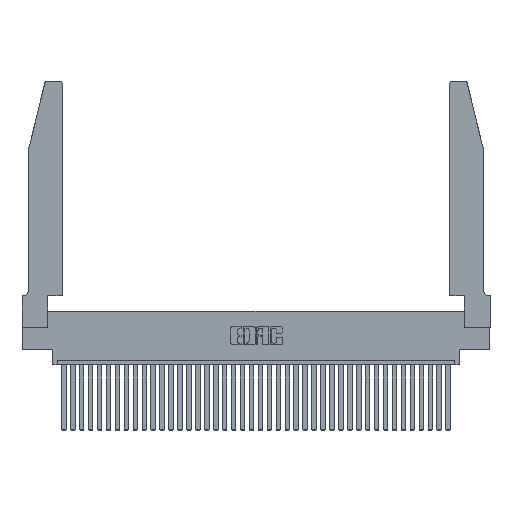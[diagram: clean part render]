
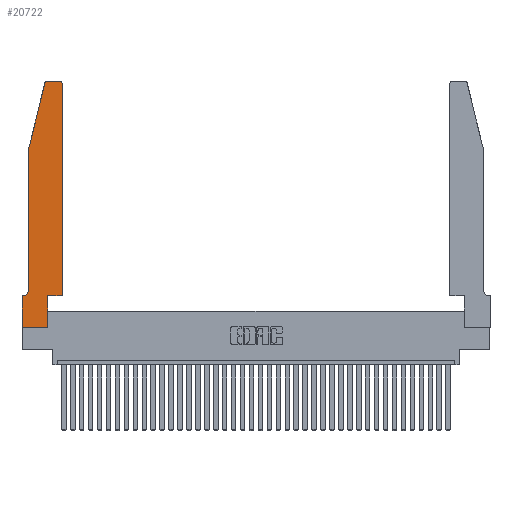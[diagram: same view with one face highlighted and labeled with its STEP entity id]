
A CAD part, top view. The second image highlights one B-rep face of the part: STEP entity #20722.
In plain terms, the highlighted planar face has unit normal (0, 0, 1).
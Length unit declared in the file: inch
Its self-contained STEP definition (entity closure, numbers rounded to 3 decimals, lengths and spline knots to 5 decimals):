
#205 = DIRECTION ( 'NONE',  ( 0., -1., 0. ) ) ;
#247 = VECTOR ( 'NONE', #18984, 39.37008 ) ;
#519 = VECTOR ( 'NONE', #31377, 39.37008 ) ;
#1791 = DIRECTION ( 'NONE',  ( 1., 0., 0. ) ) ;
#2365 = ORIENTED_EDGE ( 'NONE', *, *, #12951, .T. ) ;
#3295 = EDGE_CURVE ( 'NONE', #16624, #21802, #6180, .T. ) ;
#3690 = VERTEX_POINT ( 'NONE', #7696 ) ;
#3777 = EDGE_CURVE ( 'NONE', #16134, #16624, #28448, .T. ) ;
#4369 = ORIENTED_EDGE ( 'NONE', *, *, #4507, .T. ) ;
#4507 = EDGE_CURVE ( 'NONE', #34466, #29771, #30644, .T. ) ;
#4843 = EDGE_CURVE ( 'NONE', #34235, #20024, #15168, .T. ) ;
#5277 = DIRECTION ( 'NONE',  ( -0.239, -0.971, 0. ) ) ;
#5660 = CARTESIAN_POINT ( 'NONE',  ( 0.25487, 2.72718, 0.37 ) ) ;
#5789 = ORIENTED_EDGE ( 'NONE', *, *, #15456, .T. ) ;
#6180 = LINE ( 'NONE', #20692, #12575 ) ;
#7357 = VECTOR ( 'NONE', #10243, 39.37008 ) ;
#7696 = CARTESIAN_POINT ( 'NONE',  ( 0.2865, 0., 0.37 ) ) ;
#8141 = CARTESIAN_POINT ( 'NONE',  ( 0.4505, 0.35, 0.37 ) ) ;
#8478 = ORIENTED_EDGE ( 'NONE', *, *, #12542, .T. ) ;
#8930 = CARTESIAN_POINT ( 'NONE',  ( 0., 0.35, 0.37 ) ) ;
#8931 = ORIENTED_EDGE ( 'NONE', *, *, #23964, .T. ) ;
#9040 = DIRECTION ( 'NONE',  ( -1., 0., 0. ) ) ;
#9819 = AXIS2_PLACEMENT_3D ( 'NONE', #24844, #33517, #1791 ) ;
#9960 = CARTESIAN_POINT ( 'NONE',  ( 0.2605, 2.75, 0.37 ) ) ;
#10243 = DIRECTION ( 'NONE',  ( 1., 0., 0. ) ) ;
#10736 = VECTOR ( 'NONE', #5277, 39.37008 ) ;
#10779 = ORIENTED_EDGE ( 'NONE', *, *, #3777, .T. ) ;
#11131 = VECTOR ( 'NONE', #12914, 39.37008 ) ;
#11503 = CARTESIAN_POINT ( 'NONE',  ( 0.0755, 2., 0.37 ) ) ;
#11596 = CARTESIAN_POINT ( 'NONE',  ( 0.284, 2.75, 0.37 ) ) ;
#11915 = CARTESIAN_POINT ( 'NONE',  ( 0.2865, 0.35, 0.37 ) ) ;
#12224 = CARTESIAN_POINT ( 'NONE',  ( 0.2865, 0.35, 0.37 ) ) ;
#12542 = EDGE_CURVE ( 'NONE', #3690, #18731, #31491, .T. ) ;
#12575 = VECTOR ( 'NONE', #205, 39.37008 ) ;
#12914 = DIRECTION ( 'NONE',  ( -1., 0., 0. ) ) ;
#12951 = EDGE_CURVE ( 'NONE', #29771, #16134, #32325, .T. ) ;
#13249 = PLANE ( 'NONE',  #9819 ) ;
#13714 = CARTESIAN_POINT ( 'NONE',  ( 0.4505, 0.35, 0.37 ) ) ;
#14049 = CARTESIAN_POINT ( 'NONE',  ( 0.4205, 2.72, 0.37 ) ) ;
#14190 = DIRECTION ( 'NONE',  ( -1., 0., 0. ) ) ;
#14712 = EDGE_CURVE ( 'NONE', #20024, #32909, #15655, .T. ) ;
#15163 = CARTESIAN_POINT ( 'NONE',  ( 0.0055, 0.42, 0.37 ) ) ;
#15168 = LINE ( 'NONE', #31306, #22939 ) ;
#15279 = EDGE_CURVE ( 'NONE', #18394, #23338, #25617, .T. ) ;
#15376 = ORIENTED_EDGE ( 'NONE', *, *, #28176, .T. ) ;
#15456 = EDGE_CURVE ( 'NONE', #32909, #3690, #34580, .T. ) ;
#15525 = ORIENTED_EDGE ( 'NONE', *, *, #14712, .T. ) ;
#15542 = DIRECTION ( 'NONE',  ( 1., 0., 0. ) ) ;
#15592 = VECTOR ( 'NONE', #35778, 39.37008 ) ;
#15655 = LINE ( 'NONE', #19056, #17462 ) ;
#16134 = VERTEX_POINT ( 'NONE', #5660 ) ;
#16269 = DIRECTION ( 'NONE',  ( 0., -1., 0. ) ) ;
#16624 = VERTEX_POINT ( 'NONE', #36129 ) ;
#17462 = VECTOR ( 'NONE', #16269, 39.37008 ) ;
#17879 = AXIS2_PLACEMENT_3D ( 'NONE', #26705, #26352, #15542 ) ;
#18062 = CARTESIAN_POINT ( 'NONE',  ( 0.0755, 0.42, 0.37 ) ) ;
#18394 = VERTEX_POINT ( 'NONE', #13714 ) ;
#18650 = AXIS2_PLACEMENT_3D ( 'NONE', #14049, #28507, #25737 ) ;
#18731 = VERTEX_POINT ( 'NONE', #11915 ) ;
#18780 = CARTESIAN_POINT ( 'NONE',  ( 0., 0., 0.37 ) ) ;
#18984 = DIRECTION ( 'NONE',  ( 1., 0., 0. ) ) ;
#19056 = CARTESIAN_POINT ( 'NONE',  ( 0., 0., 0.37 ) ) ;
#20024 = VERTEX_POINT ( 'NONE', #8930 ) ;
#20692 = CARTESIAN_POINT ( 'NONE',  ( 0.0755, 2., 0.37 ) ) ;
#20722 = ADVANCED_FACE ( 'NONE', ( #31329 ), #13249, .T. ) ;
#21256 = AXIS2_PLACEMENT_3D ( 'NONE', #15163, #32630, #9040 ) ;
#21802 = VERTEX_POINT ( 'NONE', #18062 ) ;
#21854 = CIRCLE ( 'NONE', #21256, 0.07 ) ;
#22939 = VECTOR ( 'NONE', #14190, 39.37008 ) ;
#23338 = VERTEX_POINT ( 'NONE', #30937 ) ;
#23964 = EDGE_CURVE ( 'NONE', #23338, #34466, #24258, .T. ) ;
#24258 = CIRCLE ( 'NONE', #18650, 0.03 ) ;
#24424 = LINE ( 'NONE', #24580, #247 ) ;
#24580 = CARTESIAN_POINT ( 'NONE',  ( 0.4505, 0.35, 0.37 ) ) ;
#24844 = CARTESIAN_POINT ( 'NONE',  ( 0., 0.35, 0.37 ) ) ;
#25617 = LINE ( 'NONE', #8141, #519 ) ;
#25737 = DIRECTION ( 'NONE',  ( 1., 0., 0. ) ) ;
#26352 = DIRECTION ( 'NONE',  ( 0., 0., 1. ) ) ;
#26705 = CARTESIAN_POINT ( 'NONE',  ( 0.284, 2.72, 0.37 ) ) ;
#28176 = EDGE_CURVE ( 'NONE', #18731, #18394, #24424, .T. ) ;
#28448 = LINE ( 'NONE', #11503, #10736 ) ;
#28507 = DIRECTION ( 'NONE',  ( 0., 0., 1. ) ) ;
#28786 = ORIENTED_EDGE ( 'NONE', *, *, #3295, .T. ) ;
#28847 = ORIENTED_EDGE ( 'NONE', *, *, #15279, .T. ) ;
#29771 = VERTEX_POINT ( 'NONE', #11596 ) ;
#30644 = LINE ( 'NONE', #9960, #11131 ) ;
#30937 = CARTESIAN_POINT ( 'NONE',  ( 0.4505, 2.72, 0.37 ) ) ;
#31306 = CARTESIAN_POINT ( 'NONE',  ( 0.0755, 0.35, 0.37 ) ) ;
#31329 = FACE_OUTER_BOUND ( 'NONE', #32513, .T. ) ;
#31377 = DIRECTION ( 'NONE',  ( 0., 1., 0. ) ) ;
#31491 = LINE ( 'NONE', #12224, #15592 ) ;
#31968 = EDGE_CURVE ( 'NONE', #21802, #34235, #21854, .T. ) ;
#32325 = CIRCLE ( 'NONE', #17879, 0.03 ) ;
#32513 = EDGE_LOOP ( 'NONE', ( #4369, #2365, #10779, #28786, #34393, #33490, #15525, #5789, #8478, #15376, #28847, #8931 ) ) ;
#32630 = DIRECTION ( 'NONE',  ( 0., 0., -1. ) ) ;
#32909 = VERTEX_POINT ( 'NONE', #35187 ) ;
#33490 = ORIENTED_EDGE ( 'NONE', *, *, #4843, .T. ) ;
#33517 = DIRECTION ( 'NONE',  ( 0., 0., 1. ) ) ;
#34083 = CARTESIAN_POINT ( 'NONE',  ( 0.0055, 0.35, 0.37 ) ) ;
#34235 = VERTEX_POINT ( 'NONE', #34083 ) ;
#34393 = ORIENTED_EDGE ( 'NONE', *, *, #31968, .T. ) ;
#34466 = VERTEX_POINT ( 'NONE', #37450 ) ;
#34580 = LINE ( 'NONE', #18780, #7357 ) ;
#35187 = CARTESIAN_POINT ( 'NONE',  ( 0., 0., 0.37 ) ) ;
#35778 = DIRECTION ( 'NONE',  ( 0., 1., 0. ) ) ;
#36129 = CARTESIAN_POINT ( 'NONE',  ( 0.0755, 2., 0.37 ) ) ;
#37450 = CARTESIAN_POINT ( 'NONE',  ( 0.4205, 2.75, 0.37 ) ) ;
